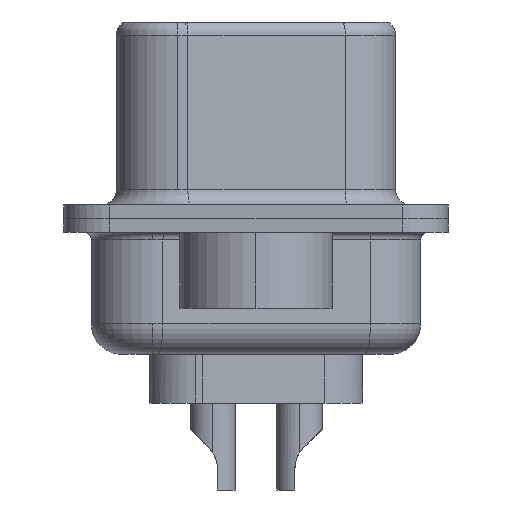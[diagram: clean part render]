
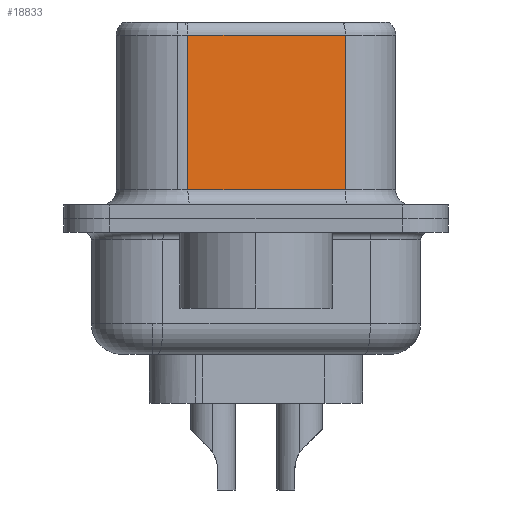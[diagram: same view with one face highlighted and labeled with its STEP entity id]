
A CAD part, left-side view. The second image highlights one B-rep face of the part: STEP entity #18833.
In plain terms, the highlighted planar face has unit normal (-0.985, -0.174, 0).
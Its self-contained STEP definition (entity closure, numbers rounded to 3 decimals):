
#1143 = LINE ( 'NONE', #3062, #18397 ) ;
#1551 = VERTEX_POINT ( 'NONE', #13321 ) ;
#2026 = LINE ( 'NONE', #4357, #20553 ) ;
#3062 = CARTESIAN_POINT ( 'NONE',  ( 4.58, -2.927, 0.95 ) ) ;
#3366 = CARTESIAN_POINT ( 'NONE',  ( 4.58, -2.927, 6.02 ) ) ;
#3586 = ORIENTED_EDGE ( 'NONE', *, *, #11315, .T. ) ;
#4357 = CARTESIAN_POINT ( 'NONE',  ( 3.67, 2.233, 6.52 ) ) ;
#4715 = ORIENTED_EDGE ( 'NONE', *, *, #12767, .F. ) ;
#7811 = CARTESIAN_POINT ( 'NONE',  ( 4.58, -2.927, 6.02 ) ) ;
#8938 = DIRECTION ( 'NONE',  ( 0., 0., -1. ) ) ;
#9481 = DIRECTION ( 'NONE',  ( 0.174, -0.985, 0. ) ) ;
#9785 = VERTEX_POINT ( 'NONE', #12237 ) ;
#11315 = EDGE_CURVE ( 'NONE', #9785, #21516, #2026, .T. ) ;
#11528 = LINE ( 'NONE', #7811, #24718 ) ;
#11681 = EDGE_LOOP ( 'NONE', ( #4715, #18299, #3586, #18596 ) ) ;
#12018 = VECTOR ( 'NONE', #8938, 1000. ) ;
#12112 = CARTESIAN_POINT ( 'NONE',  ( 3.67, 2.233, 0.95 ) ) ;
#12237 = CARTESIAN_POINT ( 'NONE',  ( 3.67, 2.233, 6.02 ) ) ;
#12767 = EDGE_CURVE ( 'NONE', #14162, #1551, #19575, .T. ) ;
#13321 = CARTESIAN_POINT ( 'NONE',  ( 4.58, -2.927, 0.95 ) ) ;
#14162 = VERTEX_POINT ( 'NONE', #3366 ) ;
#14256 = DIRECTION ( 'NONE',  ( -0.174, 0.985, 0. ) ) ;
#14529 = PLANE ( 'NONE',  #20026 ) ;
#16318 = FACE_OUTER_BOUND ( 'NONE', #11681, .T. ) ;
#16477 = EDGE_CURVE ( 'NONE', #14162, #9785, #11528, .T. ) ;
#16947 = DIRECTION ( 'NONE',  ( 0., 0., -1. ) ) ;
#18299 = ORIENTED_EDGE ( 'NONE', *, *, #16477, .T. ) ;
#18397 = VECTOR ( 'NONE', #9481, 1000. ) ;
#18596 = ORIENTED_EDGE ( 'NONE', *, *, #21884, .T. ) ;
#18608 = CARTESIAN_POINT ( 'NONE',  ( 4.58, -2.927, 6.52 ) ) ;
#18833 = ADVANCED_FACE ( 'NONE', ( #16318 ), #14529, .F. ) ;
#19318 = CARTESIAN_POINT ( 'NONE',  ( 4.58, -2.927, 6.52 ) ) ;
#19575 = LINE ( 'NONE', #19318, #12018 ) ;
#20026 = AXIS2_PLACEMENT_3D ( 'NONE', #18608, #22823, #14256 ) ;
#20553 = VECTOR ( 'NONE', #16947, 1000. ) ;
#21516 = VERTEX_POINT ( 'NONE', #12112 ) ;
#21884 = EDGE_CURVE ( 'NONE', #21516, #1551, #1143, .T. ) ;
#22411 = DIRECTION ( 'NONE',  ( -0.174, 0.985, 0. ) ) ;
#22823 = DIRECTION ( 'NONE',  ( 0.985, 0.174, 0. ) ) ;
#24718 = VECTOR ( 'NONE', #22411, 1000. ) ;
